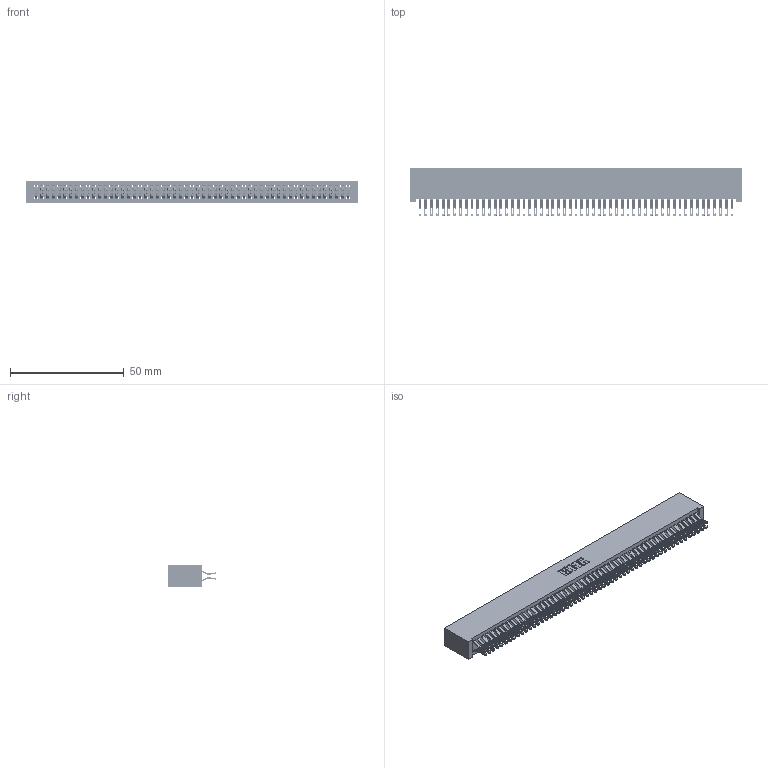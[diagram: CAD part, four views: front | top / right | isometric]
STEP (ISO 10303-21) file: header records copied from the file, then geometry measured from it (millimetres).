
FILE_DESCRIPTION (( 'STEP AP203' ), '1' );
FILE_NAME ('342-110-555-201.STEP', '2019-10-04T20:28:51', ( '' ), ( '' ), 'SwSTEP 2.0', 'SolidWorks 2016', '' );
FILE_SCHEMA (( 'CONFIG_CONTROL_DESIGN' ));
Length unit declared in the file: inch
Products named in the file (3): 342 Part_Lugless; 345-292-001_555 Tail; 342-110-555-201
Assembly tree (111 placements, depth 2):
  342-110-555-201
    342 Part_Lugless
    345-292-001_555 Tail  x110
Bounding box: 145.95 x 21.47 x 9.4 mm (x, y, z)
Volume: 13920.2 mm3; surface area: 24489.4 mm2
Topology: 111 solids, 111 shells, 6482 faces, 20405 edges, 13602 vertices
Faces by surface type: plane 3802, cylinder 2680
Entity records: 33619 total; most frequent: CARTESIAN_POINT 5588, ORIENTED_EDGE 5494, DIRECTION 4715, EDGE_CURVE 2747, VECTOR 2607, LINE 2607, VERTEX_POINT 1830, AXIS2_PLACEMENT_3D 1054
